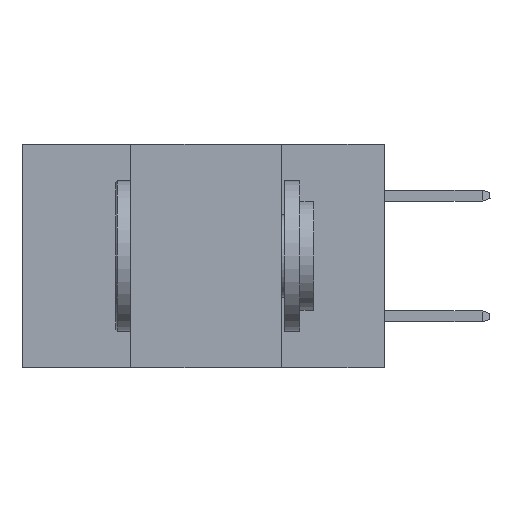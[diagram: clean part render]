
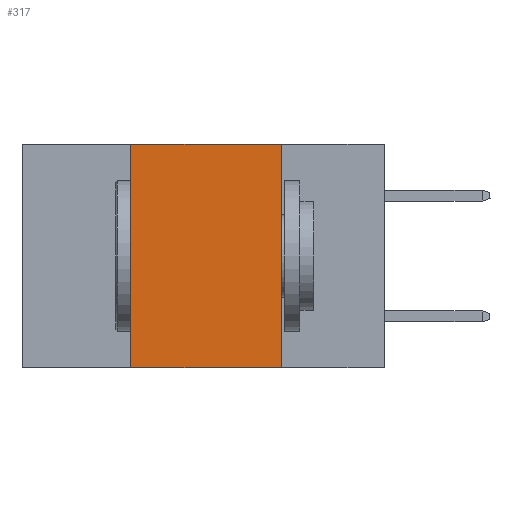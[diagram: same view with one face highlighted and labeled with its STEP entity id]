
A CAD part, left-side view. The second image highlights one B-rep face of the part: STEP entity #317.
In plain terms, the highlighted planar face has unit normal (-1, 0, 0).
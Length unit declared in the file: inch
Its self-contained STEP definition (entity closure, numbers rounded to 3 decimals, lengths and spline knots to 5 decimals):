
#301 = CARTESIAN_POINT ( 'NONE',  ( 0., 0.17, 0. ) ) ;
#317 = ADVANCED_FACE ( 'NONE', ( #11548 ), #2447, .F. ) ;
#753 = VERTEX_POINT ( 'NONE', #7198 ) ;
#1460 = CARTESIAN_POINT ( 'NONE',  ( 0., 0.42, -0.37 ) ) ;
#1618 = LINE ( 'NONE', #301, #14869 ) ;
#1623 = LINE ( 'NONE', #4276, #2832 ) ;
#1881 = CARTESIAN_POINT ( 'NONE',  ( 0., 0.6, -0.37 ) ) ;
#2146 = EDGE_CURVE ( 'NONE', #15583, #753, #9655, .T. ) ;
#2447 = PLANE ( 'NONE',  #4947 ) ;
#2585 = CARTESIAN_POINT ( 'NONE',  ( 0., 0.17, 0. ) ) ;
#2832 = VECTOR ( 'NONE', #14723, 39.37008 ) ;
#2846 = VECTOR ( 'NONE', #7080, 39.37008 ) ;
#3051 = LINE ( 'NONE', #4431, #2846 ) ;
#3119 = VERTEX_POINT ( 'NONE', #2585 ) ;
#4276 = CARTESIAN_POINT ( 'NONE',  ( 0., 0.42, 0. ) ) ;
#4431 = CARTESIAN_POINT ( 'NONE',  ( 0., 0.6, 0. ) ) ;
#4947 = AXIS2_PLACEMENT_3D ( 'NONE', #12710, #5025, #7594 ) ;
#5025 = DIRECTION ( 'NONE',  ( 1., 0., 0. ) ) ;
#5453 = DIRECTION ( 'NONE',  ( 0., 0., -1. ) ) ;
#7080 = DIRECTION ( 'NONE',  ( 0., -1., 0. ) ) ;
#7198 = CARTESIAN_POINT ( 'NONE',  ( 0., 0.17, -0.37 ) ) ;
#7594 = DIRECTION ( 'NONE',  ( 0., 0., -1. ) ) ;
#7616 = EDGE_LOOP ( 'NONE', ( #16311, #10610, #10935, #11779 ) ) ;
#7944 = EDGE_CURVE ( 'NONE', #9685, #3119, #3051, .T. ) ;
#9655 = LINE ( 'NONE', #1881, #15279 ) ;
#9685 = VERTEX_POINT ( 'NONE', #14882 ) ;
#10610 = ORIENTED_EDGE ( 'NONE', *, *, #7944, .F. ) ;
#10935 = ORIENTED_EDGE ( 'NONE', *, *, #11011, .F. ) ;
#11011 = EDGE_CURVE ( 'NONE', #15583, #9685, #1623, .T. ) ;
#11548 = FACE_OUTER_BOUND ( 'NONE', #7616, .T. ) ;
#11779 = ORIENTED_EDGE ( 'NONE', *, *, #2146, .T. ) ;
#12710 = CARTESIAN_POINT ( 'NONE',  ( 0., 0.6, 0. ) ) ;
#14224 = EDGE_CURVE ( 'NONE', #3119, #753, #1618, .T. ) ;
#14723 = DIRECTION ( 'NONE',  ( 0., 0., 1. ) ) ;
#14869 = VECTOR ( 'NONE', #5453, 39.37008 ) ;
#14882 = CARTESIAN_POINT ( 'NONE',  ( 0., 0.42, 0. ) ) ;
#15279 = VECTOR ( 'NONE', #16196, 39.37008 ) ;
#15583 = VERTEX_POINT ( 'NONE', #1460 ) ;
#16196 = DIRECTION ( 'NONE',  ( 0., -1., 0. ) ) ;
#16311 = ORIENTED_EDGE ( 'NONE', *, *, #14224, .F. ) ;
